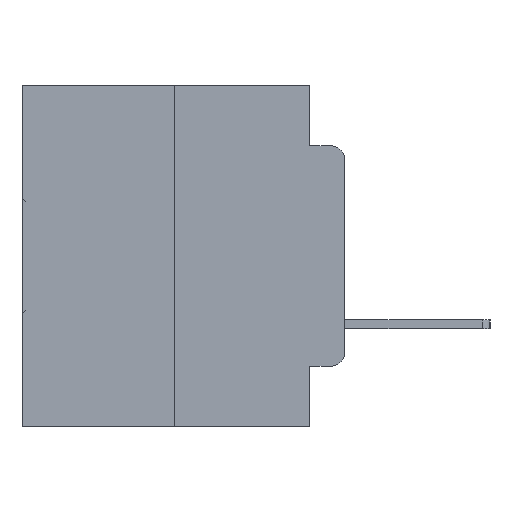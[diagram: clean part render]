
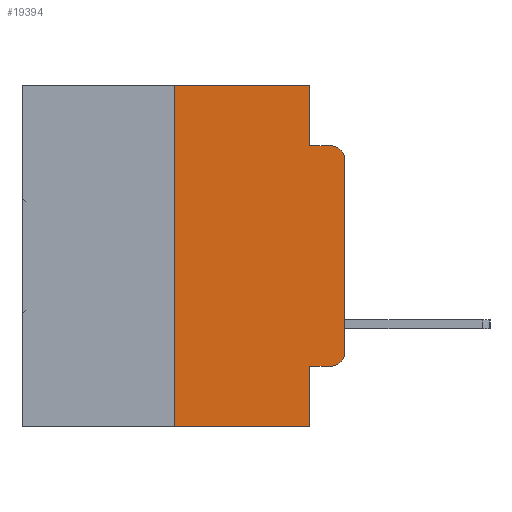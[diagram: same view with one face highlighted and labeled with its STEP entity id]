
A CAD part, left-side view. The second image highlights one B-rep face of the part: STEP entity #19394.
In plain terms, the highlighted planar face has unit normal (-1, 0, 0).
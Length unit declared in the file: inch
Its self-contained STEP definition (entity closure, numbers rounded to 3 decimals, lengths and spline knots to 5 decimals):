
#89 = LINE ( 'NONE', #12101, #5076 ) ;
#126 = EDGE_CURVE ( 'NONE', #15633, #18950, #24177, .T. ) ;
#1146 = CARTESIAN_POINT ( 'NONE',  ( 0., 0.051, -0.0885 ) ) ;
#1729 = DIRECTION ( 'NONE',  ( 0., 0., 1. ) ) ;
#1904 = DIRECTION ( 'NONE',  ( 0., 0., -1. ) ) ;
#2314 = DIRECTION ( 'NONE',  ( 0., 0., -1. ) ) ;
#2390 = DIRECTION ( 'NONE',  ( 0., 0., 1. ) ) ;
#3635 = DIRECTION ( 'NONE',  ( 0., -1., 0. ) ) ;
#3642 = VERTEX_POINT ( 'NONE', #5281 ) ;
#3846 = CIRCLE ( 'NONE', #23841, 0.02 ) ;
#3945 = VERTEX_POINT ( 'NONE', #9081 ) ;
#4429 = PLANE ( 'NONE',  #10520 ) ;
#4927 = LINE ( 'NONE', #30384, #16969 ) ;
#5023 = CARTESIAN_POINT ( 'NONE',  ( 0., 0.02, -0.3915 ) ) ;
#5076 = VECTOR ( 'NONE', #2390, 39.37008 ) ;
#5281 = CARTESIAN_POINT ( 'NONE',  ( 0., 0.25, 0. ) ) ;
#5417 = VECTOR ( 'NONE', #1904, 39.37008 ) ;
#6169 = LINE ( 'NONE', #6721, #5417 ) ;
#6244 = ORIENTED_EDGE ( 'NONE', *, *, #27437, .F. ) ;
#6721 = CARTESIAN_POINT ( 'NONE',  ( 0., 0.051, 0. ) ) ;
#7164 = VERTEX_POINT ( 'NONE', #22474 ) ;
#7484 = DIRECTION ( 'NONE',  ( 0., 0., -1. ) ) ;
#7678 = CARTESIAN_POINT ( 'NONE',  ( 0., 0.25, -0.5 ) ) ;
#8089 = DIRECTION ( 'NONE',  ( -1., 0., 0. ) ) ;
#8547 = ORIENTED_EDGE ( 'NONE', *, *, #19504, .F. ) ;
#8552 = CARTESIAN_POINT ( 'NONE',  ( 0., 0.051, -0.4115 ) ) ;
#8607 = VERTEX_POINT ( 'NONE', #8552 ) ;
#8943 = ORIENTED_EDGE ( 'NONE', *, *, #25121, .T. ) ;
#9081 = CARTESIAN_POINT ( 'NONE',  ( 0., 0.051, -0.0885 ) ) ;
#9303 = CARTESIAN_POINT ( 'NONE',  ( 0., 0.473, 0. ) ) ;
#10519 = VECTOR ( 'NONE', #27353, 39.37008 ) ;
#10520 = AXIS2_PLACEMENT_3D ( 'NONE', #9303, #25978, #11683 ) ;
#10751 = EDGE_CURVE ( 'NONE', #3642, #27491, #30727, .T. ) ;
#11683 = DIRECTION ( 'NONE',  ( 0., 0., -1. ) ) ;
#11781 = LINE ( 'NONE', #1146, #23763 ) ;
#11896 = ORIENTED_EDGE ( 'NONE', *, *, #30581, .T. ) ;
#12002 = LINE ( 'NONE', #15431, #10519 ) ;
#12101 = CARTESIAN_POINT ( 'NONE',  ( 0., 0.25, 0. ) ) ;
#12253 = LINE ( 'NONE', #30938, #30461 ) ;
#12314 = CIRCLE ( 'NONE', #12677, 0.02 ) ;
#12466 = EDGE_CURVE ( 'NONE', #18513, #27043, #4927, .T. ) ;
#12628 = ORIENTED_EDGE ( 'NONE', *, *, #25862, .F. ) ;
#12677 = AXIS2_PLACEMENT_3D ( 'NONE', #22398, #8089, #24797 ) ;
#14928 = ORIENTED_EDGE ( 'NONE', *, *, #126, .T. ) ;
#15047 = DIRECTION ( 'NONE',  ( 0., -1., 0. ) ) ;
#15431 = CARTESIAN_POINT ( 'NONE',  ( 0., 0.051, -0.4115 ) ) ;
#15633 = VERTEX_POINT ( 'NONE', #7678 ) ;
#16778 = CARTESIAN_POINT ( 'NONE',  ( 0., 0.02, -0.0885 ) ) ;
#16969 = VECTOR ( 'NONE', #1729, 39.37008 ) ;
#17510 = EDGE_CURVE ( 'NONE', #8607, #7164, #12002, .T. ) ;
#18160 = VECTOR ( 'NONE', #23805, 39.37008 ) ;
#18513 = VERTEX_POINT ( 'NONE', #29296 ) ;
#18950 = VERTEX_POINT ( 'NONE', #26211 ) ;
#19106 = CARTESIAN_POINT ( 'NONE',  ( 0., 0., -0.1085 ) ) ;
#19394 = ADVANCED_FACE ( 'NONE', ( #21616 ), #4429, .F. ) ;
#19504 = EDGE_CURVE ( 'NONE', #15633, #3642, #89, .T. ) ;
#20111 = EDGE_CURVE ( 'NONE', #8607, #18950, #6169, .T. ) ;
#20548 = CARTESIAN_POINT ( 'NONE',  ( 0., 0.051, 0. ) ) ;
#21389 = CARTESIAN_POINT ( 'NONE',  ( 0., 0.473, 0. ) ) ;
#21616 = FACE_OUTER_BOUND ( 'NONE', #25393, .T. ) ;
#21804 = DIRECTION ( 'NONE',  ( -1., 0., 0. ) ) ;
#22006 = ORIENTED_EDGE ( 'NONE', *, *, #20111, .F. ) ;
#22365 = ORIENTED_EDGE ( 'NONE', *, *, #12466, .T. ) ;
#22398 = CARTESIAN_POINT ( 'NONE',  ( 0., 0.02, -0.1085 ) ) ;
#22474 = CARTESIAN_POINT ( 'NONE',  ( 0., 0.02, -0.4115 ) ) ;
#23416 = VECTOR ( 'NONE', #15047, 39.37008 ) ;
#23763 = VECTOR ( 'NONE', #3635, 39.37008 ) ;
#23805 = DIRECTION ( 'NONE',  ( 0., -1., 0. ) ) ;
#23841 = AXIS2_PLACEMENT_3D ( 'NONE', #5023, #21804, #7484 ) ;
#24177 = LINE ( 'NONE', #30364, #23416 ) ;
#24797 = DIRECTION ( 'NONE',  ( 0., 0., -1. ) ) ;
#25121 = EDGE_CURVE ( 'NONE', #7164, #18513, #3846, .T. ) ;
#25393 = EDGE_LOOP ( 'NONE', ( #22365, #11896, #6244, #12628, #26819, #8547, #14928, #22006, #26480, #8943 ) ) ;
#25862 = EDGE_CURVE ( 'NONE', #27491, #3945, #12253, .T. ) ;
#25878 = VERTEX_POINT ( 'NONE', #16778 ) ;
#25978 = DIRECTION ( 'NONE',  ( 1., 0., 0. ) ) ;
#26211 = CARTESIAN_POINT ( 'NONE',  ( 0., 0.051, -0.5 ) ) ;
#26480 = ORIENTED_EDGE ( 'NONE', *, *, #17510, .T. ) ;
#26819 = ORIENTED_EDGE ( 'NONE', *, *, #10751, .F. ) ;
#27043 = VERTEX_POINT ( 'NONE', #19106 ) ;
#27353 = DIRECTION ( 'NONE',  ( 0., -1., 0. ) ) ;
#27437 = EDGE_CURVE ( 'NONE', #3945, #25878, #11781, .T. ) ;
#27491 = VERTEX_POINT ( 'NONE', #20548 ) ;
#29296 = CARTESIAN_POINT ( 'NONE',  ( 0., 0., -0.3915 ) ) ;
#30364 = CARTESIAN_POINT ( 'NONE',  ( 0., 0.473, -0.5 ) ) ;
#30384 = CARTESIAN_POINT ( 'NONE',  ( 0., 0., 0. ) ) ;
#30461 = VECTOR ( 'NONE', #2314, 39.37008 ) ;
#30581 = EDGE_CURVE ( 'NONE', #27043, #25878, #12314, .T. ) ;
#30727 = LINE ( 'NONE', #21389, #18160 ) ;
#30938 = CARTESIAN_POINT ( 'NONE',  ( 0., 0.051, 0. ) ) ;
